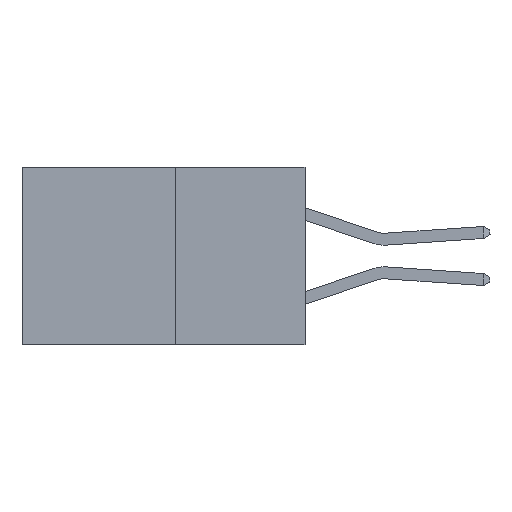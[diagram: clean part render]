
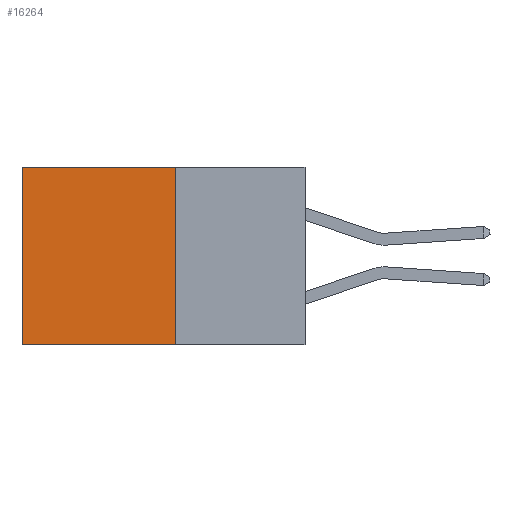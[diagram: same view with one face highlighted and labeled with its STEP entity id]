
A CAD part, left-side view. The second image highlights one B-rep face of the part: STEP entity #16264.
In plain terms, the highlighted planar face has unit normal (-1, 0, 0).
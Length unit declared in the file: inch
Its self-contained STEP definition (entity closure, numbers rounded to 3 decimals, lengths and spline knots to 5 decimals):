
#1676 = CARTESIAN_POINT ( 'NONE',  ( 0.277, 0.59, 0. ) ) ;
#1741 = ORIENTED_EDGE ( 'NONE', *, *, #16859, .T. ) ;
#2271 = EDGE_CURVE ( 'NONE', #4962, #7616, #3071, .T. ) ;
#2317 = CARTESIAN_POINT ( 'NONE',  ( 0.277, 0.27, 0. ) ) ;
#2602 = DIRECTION ( 'NONE',  ( 0., 0., -1. ) ) ;
#3071 = LINE ( 'NONE', #16521, #10201 ) ;
#3946 = LINE ( 'NONE', #10599, #11054 ) ;
#4143 = EDGE_LOOP ( 'NONE', ( #1741, #13078, #14087, #4707 ) ) ;
#4201 = CARTESIAN_POINT ( 'NONE',  ( 0.277, 0.27, -0.37 ) ) ;
#4203 = LINE ( 'NONE', #11123, #8459 ) ;
#4463 = FACE_OUTER_BOUND ( 'NONE', #4143, .T. ) ;
#4593 = CARTESIAN_POINT ( 'NONE',  ( 0.277, 0.59, -0.37 ) ) ;
#4707 = ORIENTED_EDGE ( 'NONE', *, *, #2271, .T. ) ;
#4962 = VERTEX_POINT ( 'NONE', #2317 ) ;
#5249 = VERTEX_POINT ( 'NONE', #17326 ) ;
#5360 = VECTOR ( 'NONE', #14241, 39.37008 ) ;
#5637 = DIRECTION ( 'NONE',  ( 0., 0., -1. ) ) ;
#5717 = CARTESIAN_POINT ( 'NONE',  ( 0.277, 0.27, -0.37 ) ) ;
#7616 = VERTEX_POINT ( 'NONE', #1676 ) ;
#8064 = DIRECTION ( 'NONE',  ( 0., 1., 0. ) ) ;
#8169 = EDGE_CURVE ( 'NONE', #5249, #15105, #3946, .T. ) ;
#8459 = VECTOR ( 'NONE', #2602, 39.37008 ) ;
#9081 = AXIS2_PLACEMENT_3D ( 'NONE', #4201, #14152, #5637 ) ;
#10201 = VECTOR ( 'NONE', #15416, 39.37008 ) ;
#10599 = CARTESIAN_POINT ( 'NONE',  ( 0.277, 0.27, -0.37 ) ) ;
#11054 = VECTOR ( 'NONE', #8064, 39.37008 ) ;
#11123 = CARTESIAN_POINT ( 'NONE',  ( 0.277, 0.59, -0.37 ) ) ;
#12736 = PLANE ( 'NONE',  #9081 ) ;
#12948 = LINE ( 'NONE', #5717, #5360 ) ;
#13009 = EDGE_CURVE ( 'NONE', #4962, #5249, #12948, .T. ) ;
#13078 = ORIENTED_EDGE ( 'NONE', *, *, #8169, .F. ) ;
#14087 = ORIENTED_EDGE ( 'NONE', *, *, #13009, .F. ) ;
#14152 = DIRECTION ( 'NONE',  ( 1., 0., 0. ) ) ;
#14241 = DIRECTION ( 'NONE',  ( 0., 0., -1. ) ) ;
#15105 = VERTEX_POINT ( 'NONE', #4593 ) ;
#15416 = DIRECTION ( 'NONE',  ( 0., 1., 0. ) ) ;
#16264 = ADVANCED_FACE ( 'NONE', ( #4463 ), #12736, .F. ) ;
#16521 = CARTESIAN_POINT ( 'NONE',  ( 0.277, 0.27, 0. ) ) ;
#16859 = EDGE_CURVE ( 'NONE', #7616, #15105, #4203, .T. ) ;
#17326 = CARTESIAN_POINT ( 'NONE',  ( 0.277, 0.27, -0.37 ) ) ;
